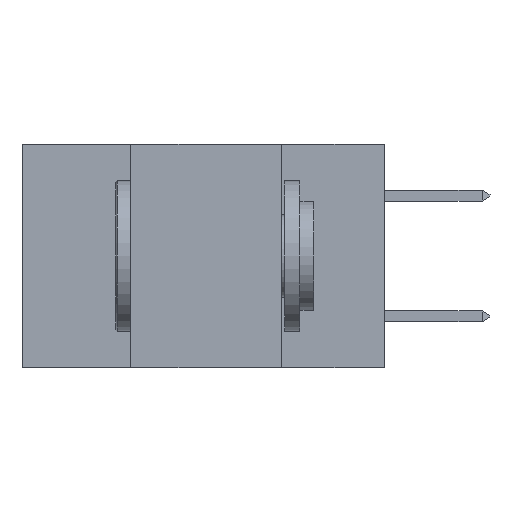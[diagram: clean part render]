
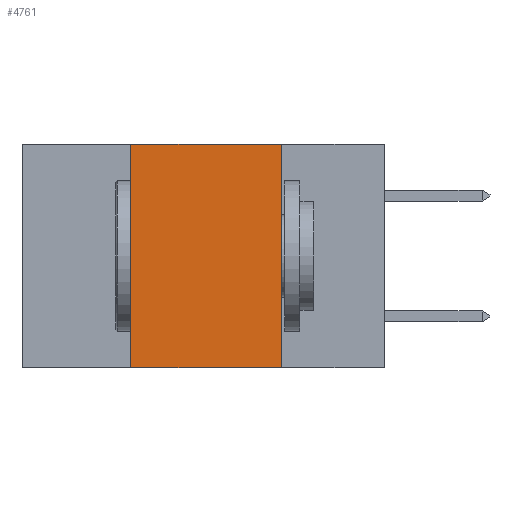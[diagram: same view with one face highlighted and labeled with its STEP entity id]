
A CAD part, left-side view. The second image highlights one B-rep face of the part: STEP entity #4761.
In plain terms, the highlighted planar face has unit normal (-1, 0, 0).
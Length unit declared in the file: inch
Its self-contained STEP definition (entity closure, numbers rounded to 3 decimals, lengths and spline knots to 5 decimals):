
#1073 = LINE ( 'NONE', #2252, #7910 ) ;
#1359 = EDGE_CURVE ( 'NONE', #1539, #7185, #4760, .T. ) ;
#1361 = VECTOR ( 'NONE', #8778, 39.37008 ) ;
#1511 = VERTEX_POINT ( 'NONE', #10207 ) ;
#1539 = VERTEX_POINT ( 'NONE', #2360 ) ;
#1856 = CARTESIAN_POINT ( 'NONE',  ( 0., 0.6, 0. ) ) ;
#1934 = CARTESIAN_POINT ( 'NONE',  ( 0., 0.6, 0. ) ) ;
#2094 = EDGE_CURVE ( 'NONE', #7185, #7467, #2596, .T. ) ;
#2252 = CARTESIAN_POINT ( 'NONE',  ( 0., 0.6, -0.37 ) ) ;
#2267 = AXIS2_PLACEMENT_3D ( 'NONE', #1934, #5308, #6863 ) ;
#2360 = CARTESIAN_POINT ( 'NONE',  ( 0., 0.42, -0.37 ) ) ;
#2596 = LINE ( 'NONE', #1856, #9818 ) ;
#3325 = DIRECTION ( 'NONE',  ( 0., -1., 0. ) ) ;
#3546 = PLANE ( 'NONE',  #2267 ) ;
#3658 = DIRECTION ( 'NONE',  ( 0., -1., 0. ) ) ;
#3957 = EDGE_CURVE ( 'NONE', #1539, #1511, #1073, .T. ) ;
#4015 = VECTOR ( 'NONE', #7961, 39.37008 ) ;
#4264 = LINE ( 'NONE', #7306, #4015 ) ;
#4760 = LINE ( 'NONE', #8040, #1361 ) ;
#4761 = ADVANCED_FACE ( 'NONE', ( #10414 ), #3546, .F. ) ;
#4855 = ORIENTED_EDGE ( 'NONE', *, *, #1359, .F. ) ;
#4936 = EDGE_LOOP ( 'NONE', ( #6812, #10204, #4855, #8643 ) ) ;
#5308 = DIRECTION ( 'NONE',  ( 1., 0., 0. ) ) ;
#6812 = ORIENTED_EDGE ( 'NONE', *, *, #7512, .F. ) ;
#6863 = DIRECTION ( 'NONE',  ( 0., 0., -1. ) ) ;
#7185 = VERTEX_POINT ( 'NONE', #8946 ) ;
#7306 = CARTESIAN_POINT ( 'NONE',  ( 0., 0.17, 0. ) ) ;
#7467 = VERTEX_POINT ( 'NONE', #8036 ) ;
#7512 = EDGE_CURVE ( 'NONE', #7467, #1511, #4264, .T. ) ;
#7910 = VECTOR ( 'NONE', #3658, 39.37008 ) ;
#7961 = DIRECTION ( 'NONE',  ( 0., 0., -1. ) ) ;
#8036 = CARTESIAN_POINT ( 'NONE',  ( 0., 0.17, 0. ) ) ;
#8040 = CARTESIAN_POINT ( 'NONE',  ( 0., 0.42, 0. ) ) ;
#8643 = ORIENTED_EDGE ( 'NONE', *, *, #3957, .T. ) ;
#8778 = DIRECTION ( 'NONE',  ( 0., 0., 1. ) ) ;
#8946 = CARTESIAN_POINT ( 'NONE',  ( 0., 0.42, 0. ) ) ;
#9818 = VECTOR ( 'NONE', #3325, 39.37008 ) ;
#10204 = ORIENTED_EDGE ( 'NONE', *, *, #2094, .F. ) ;
#10207 = CARTESIAN_POINT ( 'NONE',  ( 0., 0.17, -0.37 ) ) ;
#10414 = FACE_OUTER_BOUND ( 'NONE', #4936, .T. ) ;
